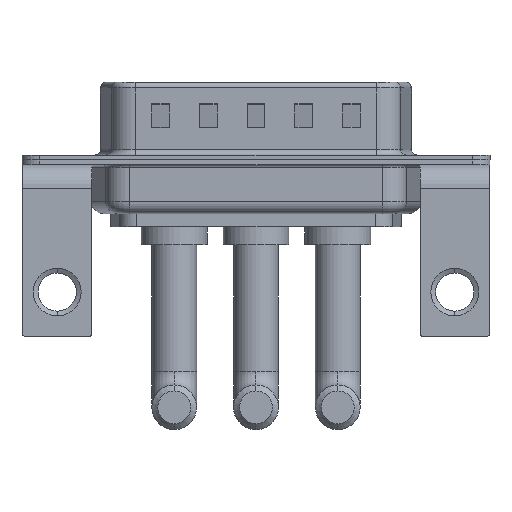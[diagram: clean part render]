
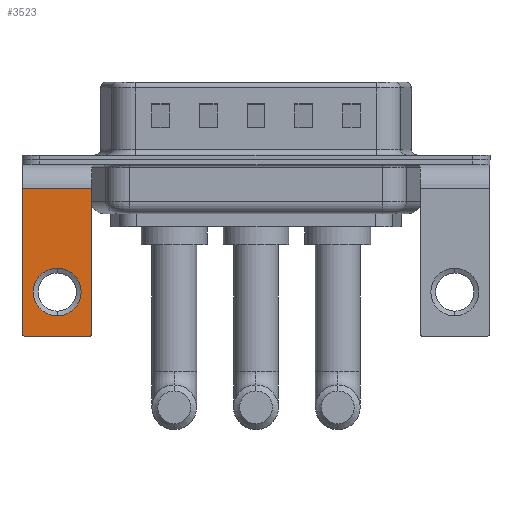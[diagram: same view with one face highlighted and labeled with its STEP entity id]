
A CAD part, front view. The second image highlights one B-rep face of the part: STEP entity #3523.
In plain terms, the highlighted planar face has unit normal (0, -1, 0).
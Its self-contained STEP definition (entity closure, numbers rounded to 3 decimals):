
#182 = CARTESIAN_POINT ( 'NONE',  ( -2.9, -6.25, -14.55 ) ) ;
#272 = ORIENTED_EDGE ( 'NONE', *, *, #9977, .T. ) ;
#280 = ORIENTED_EDGE ( 'NONE', *, *, #1286, .T. ) ;
#420 = CARTESIAN_POINT ( 'NONE',  ( -2.9, -6.25, -2.4 ) ) ;
#622 = AXIS2_PLACEMENT_3D ( 'NONE', #15941, #14766, #2075 ) ;
#978 = VERTEX_POINT ( 'NONE', #5359 ) ;
#1286 = EDGE_CURVE ( 'NONE', #978, #9364, #8973, .T. ) ;
#1529 = VERTEX_POINT ( 'NONE', #11805 ) ;
#1722 = FACE_BOUND ( 'NONE', #11766, .T. ) ;
#1935 = ORIENTED_EDGE ( 'NONE', *, *, #16483, .T. ) ;
#2075 = DIRECTION ( 'NONE',  ( 0., 0., 1. ) ) ;
#2103 = VERTEX_POINT ( 'NONE', #420 ) ;
#2181 = ORIENTED_EDGE ( 'NONE', *, *, #15980, .T. ) ;
#2219 = LINE ( 'NONE', #13566, #15800 ) ;
#2289 = DIRECTION ( 'NONE',  ( 0., -1., 0. ) ) ;
#2365 = DIRECTION ( 'NONE',  ( -1., 0., 0. ) ) ;
#2383 = DIRECTION ( 'NONE',  ( 0., 0., 1. ) ) ;
#2440 = EDGE_CURVE ( 'NONE', #3832, #16172, #12813, .T. ) ;
#2793 = CIRCLE ( 'NONE', #622, 2. ) ;
#2961 = CARTESIAN_POINT ( 'NONE',  ( -2.65, -6.25, -14.8 ) ) ;
#3523 = ADVANCED_FACE ( 'NONE', ( #1722, #4501 ), #8117, .F. ) ;
#3832 = VERTEX_POINT ( 'NONE', #182 ) ;
#4176 = DIRECTION ( 'NONE',  ( 0., 1., 0. ) ) ;
#4251 = CARTESIAN_POINT ( 'NONE',  ( 2.9, -6.25, -2.4 ) ) ;
#4350 = CARTESIAN_POINT ( 'NONE',  ( 2.9, -6.25, -2.4 ) ) ;
#4501 = FACE_OUTER_BOUND ( 'NONE', #15777, .T. ) ;
#4516 = AXIS2_PLACEMENT_3D ( 'NONE', #10098, #2289, #9847 ) ;
#5175 = EDGE_CURVE ( 'NONE', #6489, #16172, #2219, .T. ) ;
#5359 = CARTESIAN_POINT ( 'NONE',  ( 0., -6.25, -9.07 ) ) ;
#6426 = CARTESIAN_POINT ( 'NONE',  ( 2.65, -6.25, -14.55 ) ) ;
#6489 = VERTEX_POINT ( 'NONE', #10352 ) ;
#6825 = ORIENTED_EDGE ( 'NONE', *, *, #5175, .F. ) ;
#6976 = DIRECTION ( 'NONE',  ( 0., 0., -1. ) ) ;
#7059 = VECTOR ( 'NONE', #9300, 1000. ) ;
#7429 = LINE ( 'NONE', #11378, #10847 ) ;
#7612 = DIRECTION ( 'NONE',  ( 0., -1., 0. ) ) ;
#7657 = ORIENTED_EDGE ( 'NONE', *, *, #9284, .T. ) ;
#7814 = LINE ( 'NONE', #4350, #7059 ) ;
#7866 = AXIS2_PLACEMENT_3D ( 'NONE', #6426, #7612, #2383 ) ;
#8117 = PLANE ( 'NONE',  #11261 ) ;
#8973 = CIRCLE ( 'NONE', #14608, 2. ) ;
#9284 = EDGE_CURVE ( 'NONE', #2103, #3832, #15872, .T. ) ;
#9300 = DIRECTION ( 'NONE',  ( 0., 0., -1. ) ) ;
#9364 = VERTEX_POINT ( 'NONE', #15634 ) ;
#9847 = DIRECTION ( 'NONE',  ( 0., 0., 1. ) ) ;
#9948 = DIRECTION ( 'NONE',  ( 0., 1., 0. ) ) ;
#9977 = EDGE_CURVE ( 'NONE', #9364, #978, #2793, .T. ) ;
#10098 = CARTESIAN_POINT ( 'NONE',  ( -2.65, -6.25, -14.55 ) ) ;
#10352 = CARTESIAN_POINT ( 'NONE',  ( 2.65, -6.25, -14.8 ) ) ;
#10847 = VECTOR ( 'NONE', #2365, 1000. ) ;
#11068 = CARTESIAN_POINT ( 'NONE',  ( 0., -6.25, -11.07 ) ) ;
#11261 = AXIS2_PLACEMENT_3D ( 'NONE', #4251, #4176, #12130 ) ;
#11378 = CARTESIAN_POINT ( 'NONE',  ( 2.9, -6.25, -2.4 ) ) ;
#11766 = EDGE_LOOP ( 'NONE', ( #272, #280 ) ) ;
#11805 = CARTESIAN_POINT ( 'NONE',  ( 2.9, -6.25, -2.4 ) ) ;
#12130 = DIRECTION ( 'NONE',  ( 0., 0., 1. ) ) ;
#12813 = CIRCLE ( 'NONE', #4516, 0.25 ) ;
#13181 = CARTESIAN_POINT ( 'NONE',  ( -2.9, -6.25, -2.4 ) ) ;
#13494 = VECTOR ( 'NONE', #6976, 1000. ) ;
#13566 = CARTESIAN_POINT ( 'NONE',  ( 2.9, -6.25, -14.8 ) ) ;
#13645 = DIRECTION ( 'NONE',  ( -1., 0., 0. ) ) ;
#13744 = CARTESIAN_POINT ( 'NONE',  ( 2.9, -6.25, -14.55 ) ) ;
#13787 = EDGE_CURVE ( 'NONE', #1529, #15357, #7814, .T. ) ;
#13846 = ORIENTED_EDGE ( 'NONE', *, *, #2440, .T. ) ;
#14608 = AXIS2_PLACEMENT_3D ( 'NONE', #11068, #9948, #15085 ) ;
#14659 = ORIENTED_EDGE ( 'NONE', *, *, #13787, .F. ) ;
#14766 = DIRECTION ( 'NONE',  ( 0., 1., 0. ) ) ;
#15085 = DIRECTION ( 'NONE',  ( 0., 0., 1. ) ) ;
#15100 = CIRCLE ( 'NONE', #7866, 0.25 ) ;
#15357 = VERTEX_POINT ( 'NONE', #13744 ) ;
#15634 = CARTESIAN_POINT ( 'NONE',  ( 0., -6.25, -13.07 ) ) ;
#15777 = EDGE_LOOP ( 'NONE', ( #7657, #13846, #6825, #2181, #14659, #1935 ) ) ;
#15800 = VECTOR ( 'NONE', #13645, 1000. ) ;
#15872 = LINE ( 'NONE', #13181, #13494 ) ;
#15941 = CARTESIAN_POINT ( 'NONE',  ( 0., -6.25, -11.07 ) ) ;
#15980 = EDGE_CURVE ( 'NONE', #6489, #15357, #15100, .T. ) ;
#16172 = VERTEX_POINT ( 'NONE', #2961 ) ;
#16483 = EDGE_CURVE ( 'NONE', #1529, #2103, #7429, .T. ) ;
